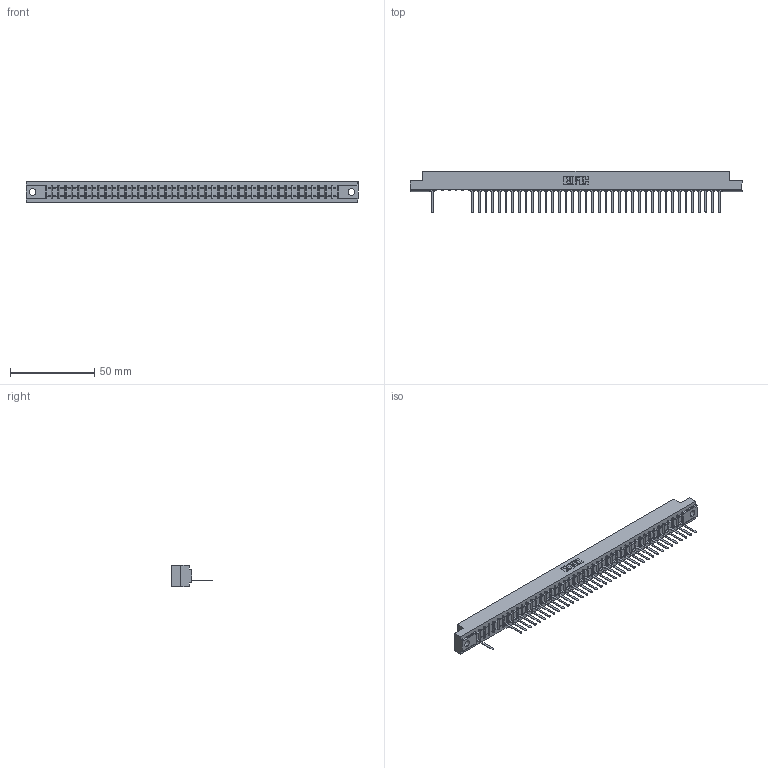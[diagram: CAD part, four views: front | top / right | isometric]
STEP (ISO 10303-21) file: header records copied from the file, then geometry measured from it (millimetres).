
FILE_DESCRIPTION (( 'STEP AP203' ), '1' );
FILE_NAME ('357-044-541-104.STEP', '2018-08-11T11:35:07', ( '' ), ( '' ), 'SwSTEP 2.0', 'SolidWorks 2016', '' );
FILE_SCHEMA (( 'CONFIG_CONTROL_DESIGN' ));
Length unit declared in the file: inch
Products named in the file (3): 307 Part_.156 Dia Mounting Holes; 307-290-002_541; 357-044-541-104
Assembly tree (40 placements, depth 2):
  357-044-541-104
    307 Part_.156 Dia Mounting Holes
    307-290-002_541  x39
Bounding box: 197.36 x 24.59 x 12.7 mm (x, y, z)
Volume: 20994.1 mm3; surface area: 26058.2 mm2
Topology: 40 solids, 40 shells, 3163 faces, 9727 edges, 6362 vertices
Faces by surface type: plane 1899, cylinder 1174, sphere 90
Entity records: 38450 total; most frequent: CARTESIAN_POINT 6513, ORIENTED_EDGE 6506, DIRECTION 6313, EDGE_CURVE 3253, LINE 2501, VECTOR 2501, VERTEX_POINT 2106, AXIS2_PLACEMENT_3D 1906
